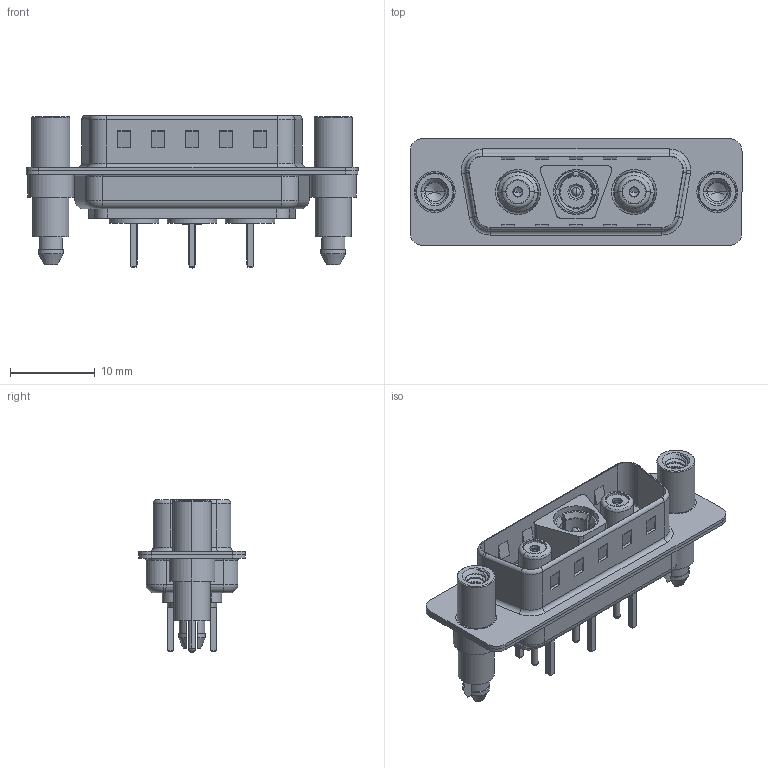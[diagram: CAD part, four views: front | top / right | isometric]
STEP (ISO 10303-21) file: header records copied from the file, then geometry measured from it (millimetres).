
FILE_DESCRIPTION (( 'STEP AP203' ), '1' );
FILE_NAME ('627-3WK3624-7N6.STEP', '2019-05-25T02:00:57', ( '' ), ( '' ), 'SwSTEP 2.0', 'SolidWorks 2016', '' );
FILE_SCHEMA (( 'CONFIG_CONTROL_DESIGN' ));
Length unit declared in the file: millimetre
Products named in the file (15): Co-Ax Jack Assy_S; Insulator Pin_Straight PC Tail; 627-3WK3624-7N6; Pin_Str; Locking Collar; Co-Ax Plug Assy_S; 627Combo Housing_3WK3; Co-Ax Jack_Straight PC Tail; 627Combo Shell Rear_15 Contacts; Insulator Socket; 627Combo Shell Front_15 Contacts; Insulator Socket 2; 627Combo Threaded Standoff and Boardlock_6; Socket_Str; Co-Ax Plug_Straight PC Tail
Assembly tree (17 placements, depth 3):
  627-3WK3624-7N6
    627Combo Housing_3WK3
    627Combo Shell Rear_15 Contacts
    627Combo Shell Front_15 Contacts
    627Combo Threaded Standoff and Boardlock_6  x2
    Co-Ax Plug Assy_S
      Co-Ax Plug_Straight PC Tail
      Insulator Pin_Straight PC Tail
      Pin_Str
      Locking Collar
    Co-Ax Jack Assy_S  x2
      Co-Ax Jack_Straight PC Tail
      Insulator Socket
      Insulator Socket 2
      Locking Collar
      Socket_Str
Bounding box: 39.15 x 12.6 x 18 mm (x, y, z)
Volume: 2354.5 mm3; surface area: 6546.9 mm2
Topology: 19 solids, 19 shells, 751 faces, 1815 edges, 1144 vertices
Faces by surface type: plane 313, cylinder 305, torus 62, cone 51, bspline 12, sphere 8
Entity records: 19852 total; most frequent: CARTESIAN_POINT 4283, DIRECTION 3055, ORIENTED_EDGE 2796, EDGE_CURVE 1398, AXIS2_PLACEMENT_3D 1155, VERTEX_POINT 889, LINE 745, VECTOR 745
